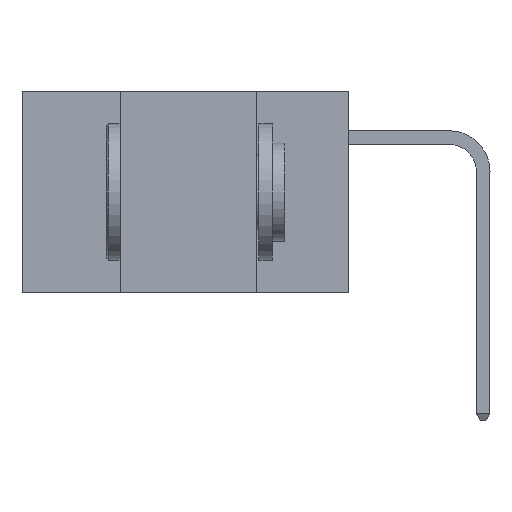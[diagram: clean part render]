
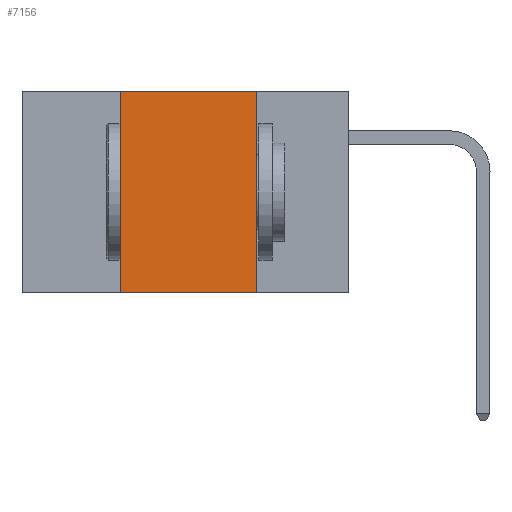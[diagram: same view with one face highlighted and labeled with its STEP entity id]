
A CAD part, left-side view. The second image highlights one B-rep face of the part: STEP entity #7156.
In plain terms, the highlighted planar face has unit normal (-1, 0, 0).
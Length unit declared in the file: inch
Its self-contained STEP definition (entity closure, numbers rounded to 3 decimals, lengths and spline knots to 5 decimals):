
#253 = FACE_OUTER_BOUND ( 'NONE', #8927, .T. ) ;
#292 = ORIENTED_EDGE ( 'NONE', *, *, #6924, .F. ) ;
#768 = CARTESIAN_POINT ( 'NONE',  ( 0., 0.17, -0.37 ) ) ;
#810 = CARTESIAN_POINT ( 'NONE',  ( 0., 0.42, 0. ) ) ;
#1124 = LINE ( 'NONE', #3033, #1312 ) ;
#1312 = VECTOR ( 'NONE', #9285, 39.37008 ) ;
#1929 = ORIENTED_EDGE ( 'NONE', *, *, #4506, .T. ) ;
#1992 = DIRECTION ( 'NONE',  ( 0., -1., 0. ) ) ;
#2088 = CARTESIAN_POINT ( 'NONE',  ( 0., 0.6, -0.37 ) ) ;
#2482 = VERTEX_POINT ( 'NONE', #810 ) ;
#3033 = CARTESIAN_POINT ( 'NONE',  ( 0., 0.42, 0. ) ) ;
#3594 = PLANE ( 'NONE',  #7466 ) ;
#4030 = DIRECTION ( 'NONE',  ( 0., 0., -1. ) ) ;
#4506 = EDGE_CURVE ( 'NONE', #5046, #4644, #10579, .T. ) ;
#4628 = DIRECTION ( 'NONE',  ( 1., 0., 0. ) ) ;
#4644 = VERTEX_POINT ( 'NONE', #768 ) ;
#4699 = CARTESIAN_POINT ( 'NONE',  ( 0., 0.6, 0. ) ) ;
#4869 = CARTESIAN_POINT ( 'NONE',  ( 0., 0.42, -0.37 ) ) ;
#5046 = VERTEX_POINT ( 'NONE', #4869 ) ;
#5274 = VECTOR ( 'NONE', #4030, 39.37008 ) ;
#5424 = LINE ( 'NONE', #6835, #5274 ) ;
#5571 = CARTESIAN_POINT ( 'NONE',  ( 0., 0.6, 0. ) ) ;
#5828 = LINE ( 'NONE', #4699, #8087 ) ;
#6413 = EDGE_CURVE ( 'NONE', #9495, #4644, #5424, .T. ) ;
#6835 = CARTESIAN_POINT ( 'NONE',  ( 0., 0.17, 0. ) ) ;
#6874 = VECTOR ( 'NONE', #1992, 39.37008 ) ;
#6924 = EDGE_CURVE ( 'NONE', #5046, #2482, #1124, .T. ) ;
#7156 = ADVANCED_FACE ( 'NONE', ( #253 ), #3594, .F. ) ;
#7466 = AXIS2_PLACEMENT_3D ( 'NONE', #5571, #4628, #10366 ) ;
#8087 = VECTOR ( 'NONE', #8904, 39.37008 ) ;
#8274 = EDGE_CURVE ( 'NONE', #2482, #9495, #5828, .T. ) ;
#8904 = DIRECTION ( 'NONE',  ( 0., -1., 0. ) ) ;
#8927 = EDGE_LOOP ( 'NONE', ( #10903, #11160, #292, #1929 ) ) ;
#9285 = DIRECTION ( 'NONE',  ( 0., 0., 1. ) ) ;
#9495 = VERTEX_POINT ( 'NONE', #11060 ) ;
#10366 = DIRECTION ( 'NONE',  ( 0., 0., -1. ) ) ;
#10579 = LINE ( 'NONE', #2088, #6874 ) ;
#10903 = ORIENTED_EDGE ( 'NONE', *, *, #6413, .F. ) ;
#11060 = CARTESIAN_POINT ( 'NONE',  ( 0., 0.17, 0. ) ) ;
#11160 = ORIENTED_EDGE ( 'NONE', *, *, #8274, .F. ) ;
